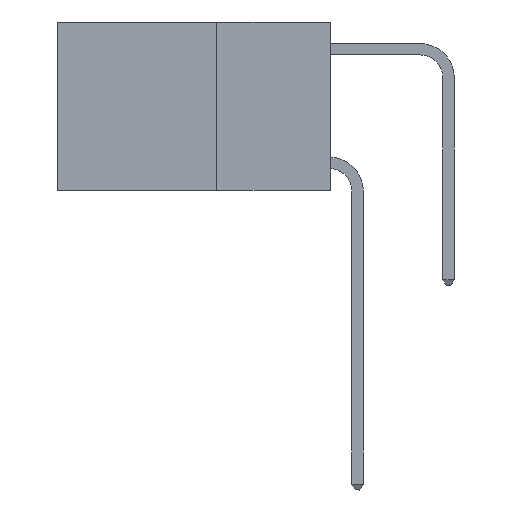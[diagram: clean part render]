
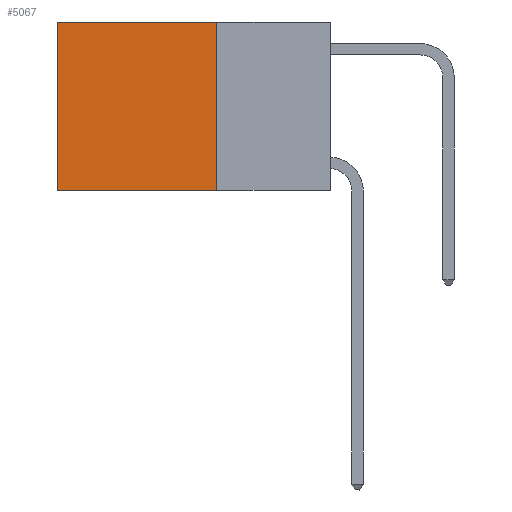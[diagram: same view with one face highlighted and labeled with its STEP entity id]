
A CAD part, left-side view. The second image highlights one B-rep face of the part: STEP entity #5067.
In plain terms, the highlighted planar face has unit normal (-1, 0, 0).
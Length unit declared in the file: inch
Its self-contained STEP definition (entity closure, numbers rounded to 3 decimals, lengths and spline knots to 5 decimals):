
#1085 = VECTOR ( 'NONE', #11937, 39.37008 ) ;
#2997 = ORIENTED_EDGE ( 'NONE', *, *, #5713, .F. ) ;
#3322 = DIRECTION ( 'NONE',  ( 0., 0., -1. ) ) ;
#3385 = EDGE_CURVE ( 'NONE', #15248, #15617, #13830, .T. ) ;
#4195 = CARTESIAN_POINT ( 'NONE',  ( 0.2625, 0.25, 0. ) ) ;
#4929 = CARTESIAN_POINT ( 'NONE',  ( 0.2625, 0.6, 0. ) ) ;
#5048 = CARTESIAN_POINT ( 'NONE',  ( 0.2625, 0.25, -0.37 ) ) ;
#5067 = ADVANCED_FACE ( 'NONE', ( #19517 ), #16032, .F. ) ;
#5713 = EDGE_CURVE ( 'NONE', #7377, #15617, #14726, .T. ) ;
#6580 = DIRECTION ( 'NONE',  ( 0., 0., -1. ) ) ;
#6600 = DIRECTION ( 'NONE',  ( 0., 1., 0. ) ) ;
#7302 = DIRECTION ( 'NONE',  ( 0., 0., -1. ) ) ;
#7377 = VERTEX_POINT ( 'NONE', #12009 ) ;
#8034 = EDGE_LOOP ( 'NONE', ( #18725, #2997, #12599, #12914 ) ) ;
#8713 = LINE ( 'NONE', #17285, #12358 ) ;
#10655 = VECTOR ( 'NONE', #3322, 39.37008 ) ;
#11046 = VERTEX_POINT ( 'NONE', #16029 ) ;
#11937 = DIRECTION ( 'NONE',  ( 0., 1., 0. ) ) ;
#12009 = CARTESIAN_POINT ( 'NONE',  ( 0.2625, 0.25, -0.37 ) ) ;
#12358 = VECTOR ( 'NONE', #6580, 39.37008 ) ;
#12447 = LINE ( 'NONE', #4195, #1085 ) ;
#12599 = ORIENTED_EDGE ( 'NONE', *, *, #18382, .F. ) ;
#12914 = ORIENTED_EDGE ( 'NONE', *, *, #16255, .T. ) ;
#13461 = CARTESIAN_POINT ( 'NONE',  ( 0.2625, 0.6, -0.37 ) ) ;
#13830 = LINE ( 'NONE', #4929, #10655 ) ;
#14532 = CARTESIAN_POINT ( 'NONE',  ( 0.2625, 0.25, 0. ) ) ;
#14726 = LINE ( 'NONE', #5048, #16192 ) ;
#15013 = DIRECTION ( 'NONE',  ( 1., 0., 0. ) ) ;
#15248 = VERTEX_POINT ( 'NONE', #16936 ) ;
#15617 = VERTEX_POINT ( 'NONE', #13461 ) ;
#16029 = CARTESIAN_POINT ( 'NONE',  ( 0.2625, 0.25, 0. ) ) ;
#16032 = PLANE ( 'NONE',  #17685 ) ;
#16192 = VECTOR ( 'NONE', #6600, 39.37008 ) ;
#16255 = EDGE_CURVE ( 'NONE', #11046, #15248, #12447, .T. ) ;
#16936 = CARTESIAN_POINT ( 'NONE',  ( 0.2625, 0.6, 0. ) ) ;
#17285 = CARTESIAN_POINT ( 'NONE',  ( 0.2625, 0.25, 0. ) ) ;
#17685 = AXIS2_PLACEMENT_3D ( 'NONE', #14532, #15013, #7302 ) ;
#18382 = EDGE_CURVE ( 'NONE', #11046, #7377, #8713, .T. ) ;
#18725 = ORIENTED_EDGE ( 'NONE', *, *, #3385, .T. ) ;
#19517 = FACE_OUTER_BOUND ( 'NONE', #8034, .T. ) ;
